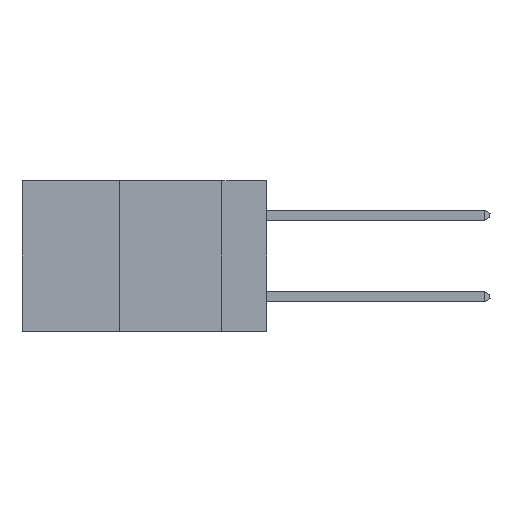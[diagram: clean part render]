
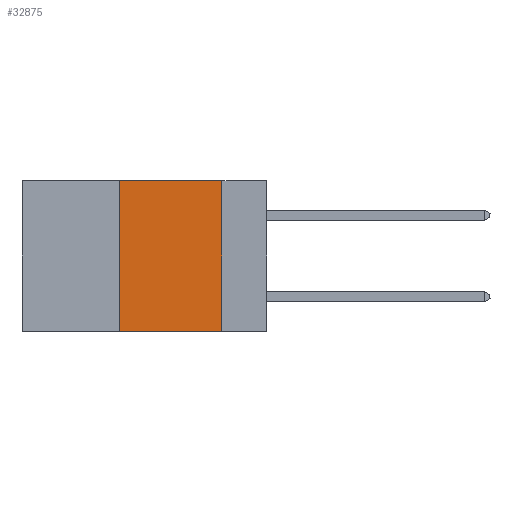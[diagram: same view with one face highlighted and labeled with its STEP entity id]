
A CAD part, left-side view. The second image highlights one B-rep face of the part: STEP entity #32875.
In plain terms, the highlighted planar face has unit normal (-1, 0, 0).
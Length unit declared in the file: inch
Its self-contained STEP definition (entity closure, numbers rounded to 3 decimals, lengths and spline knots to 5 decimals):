
#1710 = DIRECTION ( 'NONE',  ( 0., 0., -1. ) ) ;
#2585 = LINE ( 'NONE', #23433, #23245 ) ;
#2598 = VERTEX_POINT ( 'NONE', #33773 ) ;
#4007 = VECTOR ( 'NONE', #28203, 39.37008 ) ;
#4166 = ORIENTED_EDGE ( 'NONE', *, *, #22536, .F. ) ;
#7364 = LINE ( 'NONE', #27949, #4007 ) ;
#8009 = LINE ( 'NONE', #27046, #25837 ) ;
#9254 = LINE ( 'NONE', #16129, #31297 ) ;
#11825 = VERTEX_POINT ( 'NONE', #18418 ) ;
#12399 = FACE_OUTER_BOUND ( 'NONE', #12658, .T. ) ;
#12658 = EDGE_LOOP ( 'NONE', ( #4166, #27778, #33999, #22175 ) ) ;
#13703 = DIRECTION ( 'NONE',  ( 0., -1., 0. ) ) ;
#15934 = VERTEX_POINT ( 'NONE', #27316 ) ;
#16129 = CARTESIAN_POINT ( 'NONE',  ( 0., 0.11, 0. ) ) ;
#17552 = DIRECTION ( 'NONE',  ( 1., 0., 0. ) ) ;
#18418 = CARTESIAN_POINT ( 'NONE',  ( 0., 0.11, -0.37 ) ) ;
#19171 = VERTEX_POINT ( 'NONE', #31117 ) ;
#21379 = EDGE_CURVE ( 'NONE', #2598, #15934, #2585, .T. ) ;
#22175 = ORIENTED_EDGE ( 'NONE', *, *, #26202, .T. ) ;
#22536 = EDGE_CURVE ( 'NONE', #19171, #11825, #9254, .T. ) ;
#23245 = VECTOR ( 'NONE', #31024, 39.37008 ) ;
#23433 = CARTESIAN_POINT ( 'NONE',  ( 0., 0.36, 0. ) ) ;
#25323 = CARTESIAN_POINT ( 'NONE',  ( 0., 0.6, 0. ) ) ;
#25837 = VECTOR ( 'NONE', #13703, 39.37008 ) ;
#26202 = EDGE_CURVE ( 'NONE', #2598, #11825, #7364, .T. ) ;
#27046 = CARTESIAN_POINT ( 'NONE',  ( 0., 0.6, 0. ) ) ;
#27316 = CARTESIAN_POINT ( 'NONE',  ( 0., 0.36, 0. ) ) ;
#27778 = ORIENTED_EDGE ( 'NONE', *, *, #30826, .F. ) ;
#27949 = CARTESIAN_POINT ( 'NONE',  ( 0., 0.6, -0.37 ) ) ;
#28203 = DIRECTION ( 'NONE',  ( 0., -1., 0. ) ) ;
#30826 = EDGE_CURVE ( 'NONE', #15934, #19171, #8009, .T. ) ;
#31024 = DIRECTION ( 'NONE',  ( 0., 0., 1. ) ) ;
#31073 = AXIS2_PLACEMENT_3D ( 'NONE', #25323, #17552, #1710 ) ;
#31117 = CARTESIAN_POINT ( 'NONE',  ( 0., 0.11, 0. ) ) ;
#31297 = VECTOR ( 'NONE', #32203, 39.37008 ) ;
#32203 = DIRECTION ( 'NONE',  ( 0., 0., -1. ) ) ;
#32875 = ADVANCED_FACE ( 'NONE', ( #12399 ), #33469, .F. ) ;
#33469 = PLANE ( 'NONE',  #31073 ) ;
#33773 = CARTESIAN_POINT ( 'NONE',  ( 0., 0.36, -0.37 ) ) ;
#33999 = ORIENTED_EDGE ( 'NONE', *, *, #21379, .F. ) ;
